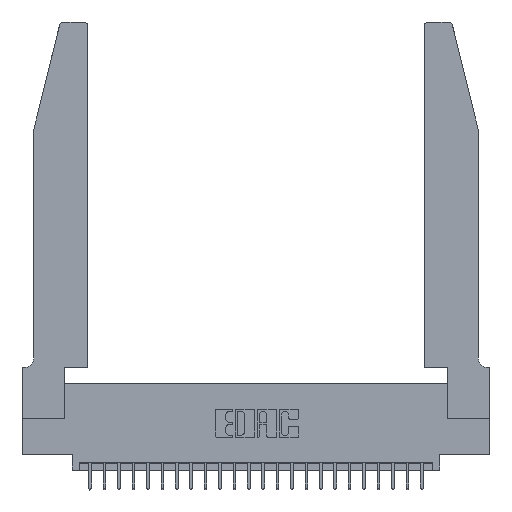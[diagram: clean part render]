
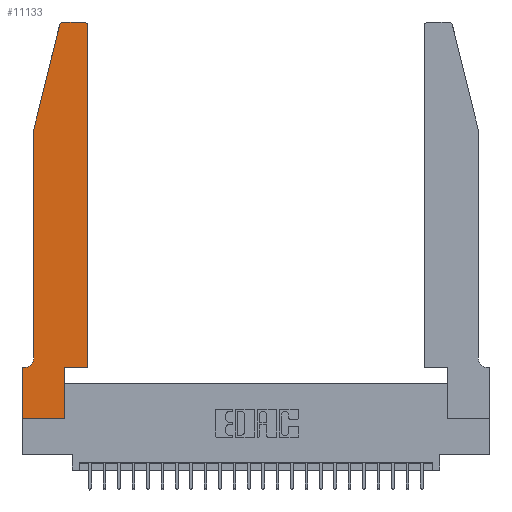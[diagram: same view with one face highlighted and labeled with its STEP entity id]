
A CAD part, top view. The second image highlights one B-rep face of the part: STEP entity #11133.
In plain terms, the highlighted planar face has unit normal (0, 0, 1).
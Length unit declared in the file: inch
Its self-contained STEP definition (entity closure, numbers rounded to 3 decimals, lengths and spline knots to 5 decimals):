
#286 = DIRECTION ( 'NONE',  ( 0., 0., 1. ) ) ;
#300 = EDGE_CURVE ( 'NONE', #22196, #1485, #20662, .T. ) ;
#585 = CARTESIAN_POINT ( 'NONE',  ( 0.2865, 0., 0.37 ) ) ;
#1303 = ORIENTED_EDGE ( 'NONE', *, *, #6294, .T. ) ;
#1485 = VERTEX_POINT ( 'NONE', #10040 ) ;
#1583 = EDGE_CURVE ( 'NONE', #16575, #20974, #13319, .T. ) ;
#1697 = ORIENTED_EDGE ( 'NONE', *, *, #24939, .T. ) ;
#1963 = DIRECTION ( 'NONE',  ( 1., 0., 0. ) ) ;
#2006 = FACE_OUTER_BOUND ( 'NONE', #7580, .T. ) ;
#2036 = DIRECTION ( 'NONE',  ( -1., 0., 0. ) ) ;
#2072 = CARTESIAN_POINT ( 'NONE',  ( 0., 0., 0.37 ) ) ;
#2158 = VERTEX_POINT ( 'NONE', #9213 ) ;
#2177 = CARTESIAN_POINT ( 'NONE',  ( 0.0055, 0.42, 0.37 ) ) ;
#2212 = VECTOR ( 'NONE', #23184, 39.37008 ) ;
#2301 = DIRECTION ( 'NONE',  ( -0.239, -0.971, 0. ) ) ;
#2533 = VERTEX_POINT ( 'NONE', #3667 ) ;
#2688 = VERTEX_POINT ( 'NONE', #19045 ) ;
#2714 = ORIENTED_EDGE ( 'NONE', *, *, #1583, .T. ) ;
#3180 = EDGE_CURVE ( 'NONE', #14788, #9190, #9683, .T. ) ;
#3445 = ORIENTED_EDGE ( 'NONE', *, *, #18823, .T. ) ;
#3651 = VERTEX_POINT ( 'NONE', #4698 ) ;
#3667 = CARTESIAN_POINT ( 'NONE',  ( 0.0755, 0.42, 0.37 ) ) ;
#4044 = CARTESIAN_POINT ( 'NONE',  ( 0., 0.35, 0.37 ) ) ;
#4139 = LINE ( 'NONE', #8005, #19482 ) ;
#4407 = CARTESIAN_POINT ( 'NONE',  ( 0.4505, 0.35, 0.37 ) ) ;
#4698 = CARTESIAN_POINT ( 'NONE',  ( 0.0055, 0.35, 0.37 ) ) ;
#4701 = CARTESIAN_POINT ( 'NONE',  ( 0.4505, 2.72, 0.37 ) ) ;
#5285 = AXIS2_PLACEMENT_3D ( 'NONE', #4044, #286, #12287 ) ;
#5400 = CARTESIAN_POINT ( 'NONE',  ( 0.0755, 0.35, 0.37 ) ) ;
#5802 = DIRECTION ( 'NONE',  ( -1., 0., 0. ) ) ;
#5878 = CARTESIAN_POINT ( 'NONE',  ( 0.284, 2.75, 0.37 ) ) ;
#6294 = EDGE_CURVE ( 'NONE', #2533, #3651, #19193, .T. ) ;
#6855 = VECTOR ( 'NONE', #16856, 39.37008 ) ;
#7041 = AXIS2_PLACEMENT_3D ( 'NONE', #13320, #21384, #20993 ) ;
#7580 = EDGE_LOOP ( 'NONE', ( #20757, #21956, #21809, #17090, #1303, #10028, #11844, #2714, #3445, #20191, #18270, #1697 ) ) ;
#8005 = CARTESIAN_POINT ( 'NONE',  ( 0., 0., 0.37 ) ) ;
#8687 = EDGE_CURVE ( 'NONE', #3651, #18281, #20558, .T. ) ;
#8894 = EDGE_CURVE ( 'NONE', #2158, #22196, #24119, .T. ) ;
#9154 = CIRCLE ( 'NONE', #7041, 0.03 ) ;
#9190 = VERTEX_POINT ( 'NONE', #4407 ) ;
#9213 = CARTESIAN_POINT ( 'NONE',  ( 0.4205, 2.75, 0.37 ) ) ;
#9683 = LINE ( 'NONE', #17765, #12754 ) ;
#9844 = VERTEX_POINT ( 'NONE', #4701 ) ;
#10028 = ORIENTED_EDGE ( 'NONE', *, *, #8687, .T. ) ;
#10040 = CARTESIAN_POINT ( 'NONE',  ( 0.25487, 2.72718, 0.37 ) ) ;
#10059 = CARTESIAN_POINT ( 'NONE',  ( 0.2605, 2.75, 0.37 ) ) ;
#10171 = CARTESIAN_POINT ( 'NONE',  ( 0.0755, 2., 0.37 ) ) ;
#11133 = ADVANCED_FACE ( 'NONE', ( #2006 ), #14511, .T. ) ;
#11427 = DIRECTION ( 'NONE',  ( 1., 0., 0. ) ) ;
#11844 = ORIENTED_EDGE ( 'NONE', *, *, #16770, .T. ) ;
#11847 = LINE ( 'NONE', #19918, #15742 ) ;
#12110 = DIRECTION ( 'NONE',  ( 0., 0., 1. ) ) ;
#12287 = DIRECTION ( 'NONE',  ( 1., 0., 0. ) ) ;
#12379 = VECTOR ( 'NONE', #22098, 39.37008 ) ;
#12579 = CARTESIAN_POINT ( 'NONE',  ( 0.0755, 2., 0.37 ) ) ;
#12754 = VECTOR ( 'NONE', #11427, 39.37008 ) ;
#12890 = VECTOR ( 'NONE', #5802, 39.37008 ) ;
#13319 = LINE ( 'NONE', #15275, #19432 ) ;
#13320 = CARTESIAN_POINT ( 'NONE',  ( 0.4205, 2.72, 0.37 ) ) ;
#14334 = DIRECTION ( 'NONE',  ( 1., 0., 0. ) ) ;
#14360 = DIRECTION ( 'NONE',  ( 0., -1., 0. ) ) ;
#14511 = PLANE ( 'NONE',  #5285 ) ;
#14762 = LINE ( 'NONE', #22831, #6855 ) ;
#14788 = VERTEX_POINT ( 'NONE', #19471 ) ;
#15275 = CARTESIAN_POINT ( 'NONE',  ( 0., 0., 0.37 ) ) ;
#15468 = VECTOR ( 'NONE', #2301, 39.37008 ) ;
#15742 = VECTOR ( 'NONE', #20578, 39.37008 ) ;
#16378 = LINE ( 'NONE', #12579, #15468 ) ;
#16417 = AXIS2_PLACEMENT_3D ( 'NONE', #24422, #12110, #14334 ) ;
#16575 = VERTEX_POINT ( 'NONE', #2072 ) ;
#16770 = EDGE_CURVE ( 'NONE', #18281, #16575, #4139, .T. ) ;
#16856 = DIRECTION ( 'NONE',  ( 0., 1., 0. ) ) ;
#17051 = AXIS2_PLACEMENT_3D ( 'NONE', #2177, #24238, #2036 ) ;
#17090 = ORIENTED_EDGE ( 'NONE', *, *, #25312, .T. ) ;
#17765 = CARTESIAN_POINT ( 'NONE',  ( 0.4505, 0.35, 0.37 ) ) ;
#18270 = ORIENTED_EDGE ( 'NONE', *, *, #25778, .T. ) ;
#18281 = VERTEX_POINT ( 'NONE', #26101 ) ;
#18823 = EDGE_CURVE ( 'NONE', #20974, #14788, #11847, .T. ) ;
#19045 = CARTESIAN_POINT ( 'NONE',  ( 0.0755, 2., 0.37 ) ) ;
#19193 = CIRCLE ( 'NONE', #17051, 0.07 ) ;
#19432 = VECTOR ( 'NONE', #1963, 39.37008 ) ;
#19471 = CARTESIAN_POINT ( 'NONE',  ( 0.2865, 0.35, 0.37 ) ) ;
#19482 = VECTOR ( 'NONE', #14360, 39.37008 ) ;
#19918 = CARTESIAN_POINT ( 'NONE',  ( 0.2865, 0.35, 0.37 ) ) ;
#20191 = ORIENTED_EDGE ( 'NONE', *, *, #3180, .T. ) ;
#20558 = LINE ( 'NONE', #5400, #2212 ) ;
#20578 = DIRECTION ( 'NONE',  ( 0., 1., 0. ) ) ;
#20662 = CIRCLE ( 'NONE', #16417, 0.03 ) ;
#20757 = ORIENTED_EDGE ( 'NONE', *, *, #8894, .T. ) ;
#20974 = VERTEX_POINT ( 'NONE', #585 ) ;
#20993 = DIRECTION ( 'NONE',  ( 1., 0., 0. ) ) ;
#21384 = DIRECTION ( 'NONE',  ( 0., 0., 1. ) ) ;
#21809 = ORIENTED_EDGE ( 'NONE', *, *, #24069, .T. ) ;
#21956 = ORIENTED_EDGE ( 'NONE', *, *, #300, .T. ) ;
#22098 = DIRECTION ( 'NONE',  ( 0., -1., 0. ) ) ;
#22196 = VERTEX_POINT ( 'NONE', #5878 ) ;
#22831 = CARTESIAN_POINT ( 'NONE',  ( 0.4505, 0.35, 0.37 ) ) ;
#23184 = DIRECTION ( 'NONE',  ( -1., 0., 0. ) ) ;
#23963 = LINE ( 'NONE', #10171, #12379 ) ;
#24069 = EDGE_CURVE ( 'NONE', #1485, #2688, #16378, .T. ) ;
#24119 = LINE ( 'NONE', #10059, #12890 ) ;
#24238 = DIRECTION ( 'NONE',  ( 0., 0., -1. ) ) ;
#24422 = CARTESIAN_POINT ( 'NONE',  ( 0.284, 2.72, 0.37 ) ) ;
#24939 = EDGE_CURVE ( 'NONE', #9844, #2158, #9154, .T. ) ;
#25312 = EDGE_CURVE ( 'NONE', #2688, #2533, #23963, .T. ) ;
#25778 = EDGE_CURVE ( 'NONE', #9190, #9844, #14762, .T. ) ;
#26101 = CARTESIAN_POINT ( 'NONE',  ( 0., 0.35, 0.37 ) ) ;
